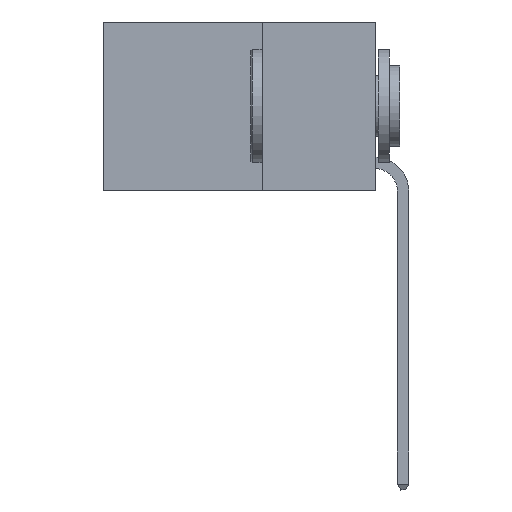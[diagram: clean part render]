
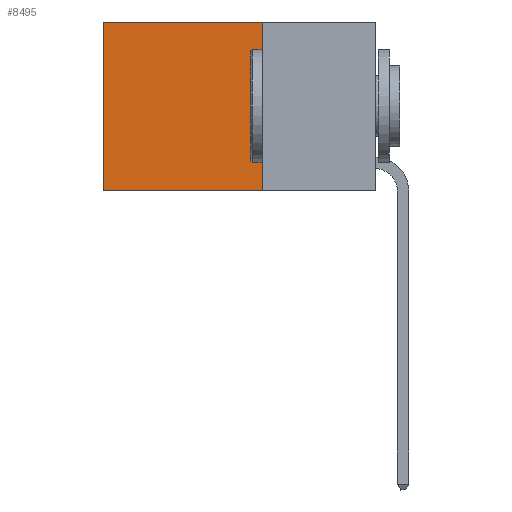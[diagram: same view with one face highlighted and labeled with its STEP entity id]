
A CAD part, left-side view. The second image highlights one B-rep face of the part: STEP entity #8495.
In plain terms, the highlighted planar face has unit normal (-1, 0, 0).
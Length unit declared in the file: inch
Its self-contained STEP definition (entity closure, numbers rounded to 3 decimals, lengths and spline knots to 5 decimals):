
#364 = CARTESIAN_POINT ( 'NONE',  ( 0.2625, 0.25, 0. ) ) ;
#901 = VECTOR ( 'NONE', #11997, 39.37008 ) ;
#1838 = DIRECTION ( 'NONE',  ( 0., 1., 0. ) ) ;
#3264 = ORIENTED_EDGE ( 'NONE', *, *, #14907, .T. ) ;
#3400 = VERTEX_POINT ( 'NONE', #10437 ) ;
#4349 = DIRECTION ( 'NONE',  ( 0., 0., -1. ) ) ;
#4613 = EDGE_CURVE ( 'NONE', #18374, #5836, #14977, .T. ) ;
#5119 = CARTESIAN_POINT ( 'NONE',  ( 0.2625, 0.25, -0.37 ) ) ;
#5130 = VERTEX_POINT ( 'NONE', #19812 ) ;
#5836 = VERTEX_POINT ( 'NONE', #8229 ) ;
#6248 = PLANE ( 'NONE',  #9176 ) ;
#7588 = ORIENTED_EDGE ( 'NONE', *, *, #18548, .T. ) ;
#7810 = VECTOR ( 'NONE', #13610, 39.37008 ) ;
#8229 = CARTESIAN_POINT ( 'NONE',  ( 0.2625, 0.25, -0.37 ) ) ;
#8495 = ADVANCED_FACE ( 'NONE', ( #18361 ), #6248, .F. ) ;
#8747 = EDGE_CURVE ( 'NONE', #5836, #3400, #20621, .T. ) ;
#9176 = AXIS2_PLACEMENT_3D ( 'NONE', #13263, #20183, #4349 ) ;
#9894 = CARTESIAN_POINT ( 'NONE',  ( 0.2625, 0.25, 0. ) ) ;
#10437 = CARTESIAN_POINT ( 'NONE',  ( 0.2625, 0.6, -0.37 ) ) ;
#10600 = LINE ( 'NONE', #12070, #11197 ) ;
#11197 = VECTOR ( 'NONE', #13999, 39.37008 ) ;
#11997 = DIRECTION ( 'NONE',  ( 0., 1., 0. ) ) ;
#12070 = CARTESIAN_POINT ( 'NONE',  ( 0.2625, 0.6, 0. ) ) ;
#13263 = CARTESIAN_POINT ( 'NONE',  ( 0.2625, 0.25, 0. ) ) ;
#13610 = DIRECTION ( 'NONE',  ( 0., 0., -1. ) ) ;
#13745 = ORIENTED_EDGE ( 'NONE', *, *, #4613, .F. ) ;
#13999 = DIRECTION ( 'NONE',  ( 0., 0., -1. ) ) ;
#14907 = EDGE_CURVE ( 'NONE', #18374, #5130, #20852, .T. ) ;
#14977 = LINE ( 'NONE', #9894, #7810 ) ;
#15443 = EDGE_LOOP ( 'NONE', ( #7588, #18654, #13745, #3264 ) ) ;
#18361 = FACE_OUTER_BOUND ( 'NONE', #15443, .T. ) ;
#18374 = VERTEX_POINT ( 'NONE', #21728 ) ;
#18548 = EDGE_CURVE ( 'NONE', #5130, #3400, #10600, .T. ) ;
#18654 = ORIENTED_EDGE ( 'NONE', *, *, #8747, .F. ) ;
#19812 = CARTESIAN_POINT ( 'NONE',  ( 0.2625, 0.6, 0. ) ) ;
#20183 = DIRECTION ( 'NONE',  ( 1., 0., 0. ) ) ;
#20621 = LINE ( 'NONE', #5119, #901 ) ;
#20852 = LINE ( 'NONE', #364, #22363 ) ;
#21728 = CARTESIAN_POINT ( 'NONE',  ( 0.2625, 0.25, 0. ) ) ;
#22363 = VECTOR ( 'NONE', #1838, 39.37008 ) ;
